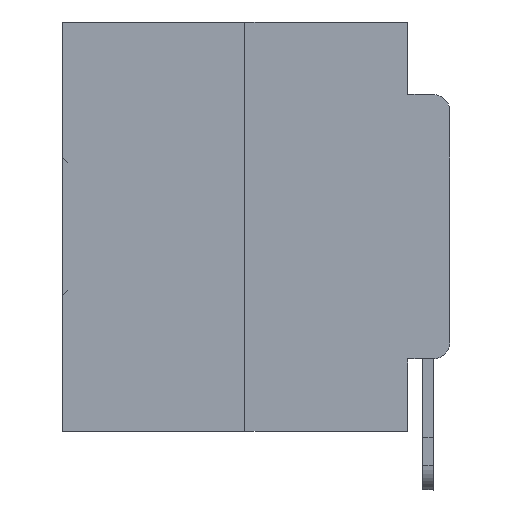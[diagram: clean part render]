
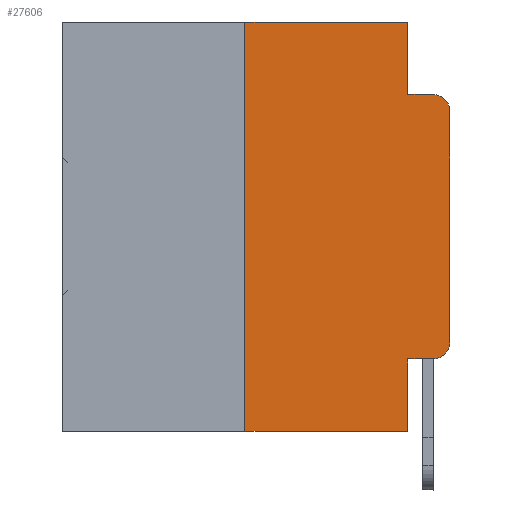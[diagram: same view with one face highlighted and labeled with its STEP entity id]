
A CAD part, left-side view. The second image highlights one B-rep face of the part: STEP entity #27606.
In plain terms, the highlighted planar face has unit normal (-1, 0, 0).
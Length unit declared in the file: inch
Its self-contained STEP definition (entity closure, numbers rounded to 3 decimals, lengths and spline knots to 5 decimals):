
#141 = VECTOR ( 'NONE', #23862, 39.37008 ) ;
#865 = DIRECTION ( 'NONE',  ( 0., 0., -1. ) ) ;
#1209 = DIRECTION ( 'NONE',  ( -1., 0., 0. ) ) ;
#1363 = CIRCLE ( 'NONE', #23575, 0.02 ) ;
#1619 = CARTESIAN_POINT ( 'NONE',  ( 0., 0.051, -0.0885 ) ) ;
#1834 = CIRCLE ( 'NONE', #33143, 0.02 ) ;
#2129 = CARTESIAN_POINT ( 'NONE',  ( 0., 0., 0. ) ) ;
#2879 = CARTESIAN_POINT ( 'NONE',  ( 0., 0.051, -0.4115 ) ) ;
#3120 = DIRECTION ( 'NONE',  ( 0., 0., -1. ) ) ;
#3246 = CARTESIAN_POINT ( 'NONE',  ( 0., 0.051, -0.0885 ) ) ;
#3296 = CARTESIAN_POINT ( 'NONE',  ( 0., 0.051, 0. ) ) ;
#3659 = ORIENTED_EDGE ( 'NONE', *, *, #18028, .T. ) ;
#4959 = CARTESIAN_POINT ( 'NONE',  ( 0., 0.473, 0. ) ) ;
#5288 = VERTEX_POINT ( 'NONE', #21463 ) ;
#6459 = DIRECTION ( 'NONE',  ( 0., 0., -1. ) ) ;
#7789 = CARTESIAN_POINT ( 'NONE',  ( 0., 0., -0.3915 ) ) ;
#7811 = DIRECTION ( 'NONE',  ( 0., -1., 0. ) ) ;
#8463 = CARTESIAN_POINT ( 'NONE',  ( 0., 0.02, -0.1085 ) ) ;
#8657 = CARTESIAN_POINT ( 'NONE',  ( 0., 0.051, 0. ) ) ;
#9633 = EDGE_CURVE ( 'NONE', #25301, #13045, #17312, .T. ) ;
#9908 = VERTEX_POINT ( 'NONE', #2879 ) ;
#10142 = LINE ( 'NONE', #4959, #20189 ) ;
#10471 = ORIENTED_EDGE ( 'NONE', *, *, #30483, .T. ) ;
#10658 = DIRECTION ( 'NONE',  ( 0., 0., -1. ) ) ;
#10670 = VERTEX_POINT ( 'NONE', #12458 ) ;
#10881 = CARTESIAN_POINT ( 'NONE',  ( 0., 0.02, -0.4115 ) ) ;
#12458 = CARTESIAN_POINT ( 'NONE',  ( 0., 0.051, -0.5 ) ) ;
#12841 = CARTESIAN_POINT ( 'NONE',  ( 0., 0.473, -0.5 ) ) ;
#13045 = VERTEX_POINT ( 'NONE', #3246 ) ;
#13111 = VECTOR ( 'NONE', #34380, 39.37008 ) ;
#13799 = VERTEX_POINT ( 'NONE', #24389 ) ;
#14133 = VECTOR ( 'NONE', #6459, 39.37008 ) ;
#14372 = LINE ( 'NONE', #17373, #21502 ) ;
#15102 = PLANE ( 'NONE',  #28408 ) ;
#15560 = EDGE_CURVE ( 'NONE', #17099, #33719, #1363, .T. ) ;
#15629 = DIRECTION ( 'NONE',  ( 1., 0., 0. ) ) ;
#15761 = CARTESIAN_POINT ( 'NONE',  ( 0., 0., -0.1085 ) ) ;
#15958 = ORIENTED_EDGE ( 'NONE', *, *, #29624, .F. ) ;
#17099 = VERTEX_POINT ( 'NONE', #15761 ) ;
#17312 = LINE ( 'NONE', #25520, #14133 ) ;
#17341 = EDGE_LOOP ( 'NONE', ( #35216, #27452, #32377, #30621, #17968, #20952, #10471, #15958, #3659, #30304 ) ) ;
#17373 = CARTESIAN_POINT ( 'NONE',  ( 0., 0.051, -0.4115 ) ) ;
#17394 = EDGE_CURVE ( 'NONE', #5288, #13799, #29043, .T. ) ;
#17822 = DIRECTION ( 'NONE',  ( 0., 0., 1. ) ) ;
#17968 = ORIENTED_EDGE ( 'NONE', *, *, #34623, .F. ) ;
#18028 = EDGE_CURVE ( 'NONE', #9908, #21316, #14372, .T. ) ;
#18310 = CARTESIAN_POINT ( 'NONE',  ( 0., 0.473, 0. ) ) ;
#19502 = LINE ( 'NONE', #3296, #29674 ) ;
#19892 = EDGE_CURVE ( 'NONE', #27723, #17099, #23333, .T. ) ;
#19914 = CARTESIAN_POINT ( 'NONE',  ( 0., 0.02, -0.3915 ) ) ;
#20189 = VECTOR ( 'NONE', #7811, 39.37008 ) ;
#20838 = CARTESIAN_POINT ( 'NONE',  ( 0., 0.25, 0. ) ) ;
#20952 = ORIENTED_EDGE ( 'NONE', *, *, #17394, .F. ) ;
#21316 = VERTEX_POINT ( 'NONE', #10881 ) ;
#21463 = CARTESIAN_POINT ( 'NONE',  ( 0., 0.25, -0.5 ) ) ;
#21502 = VECTOR ( 'NONE', #33086, 39.37008 ) ;
#22101 = VECTOR ( 'NONE', #17822, 39.37008 ) ;
#22741 = EDGE_CURVE ( 'NONE', #21316, #27723, #1834, .T. ) ;
#22992 = VECTOR ( 'NONE', #23175, 39.37008 ) ;
#23175 = DIRECTION ( 'NONE',  ( 0., -1., 0. ) ) ;
#23333 = LINE ( 'NONE', #2129, #13111 ) ;
#23575 = AXIS2_PLACEMENT_3D ( 'NONE', #8463, #30193, #27524 ) ;
#23685 = LINE ( 'NONE', #12841, #141 ) ;
#23862 = DIRECTION ( 'NONE',  ( 0., -1., 0. ) ) ;
#24389 = CARTESIAN_POINT ( 'NONE',  ( 0., 0.25, 0. ) ) ;
#25301 = VERTEX_POINT ( 'NONE', #8657 ) ;
#25520 = CARTESIAN_POINT ( 'NONE',  ( 0., 0.051, 0. ) ) ;
#27452 = ORIENTED_EDGE ( 'NONE', *, *, #15560, .T. ) ;
#27524 = DIRECTION ( 'NONE',  ( 0., 0., -1. ) ) ;
#27606 = ADVANCED_FACE ( 'NONE', ( #31861 ), #15102, .F. ) ;
#27723 = VERTEX_POINT ( 'NONE', #7789 ) ;
#28408 = AXIS2_PLACEMENT_3D ( 'NONE', #18310, #15629, #10658 ) ;
#29043 = LINE ( 'NONE', #20838, #22101 ) ;
#29624 = EDGE_CURVE ( 'NONE', #9908, #10670, #19502, .T. ) ;
#29674 = VECTOR ( 'NONE', #3120, 39.37008 ) ;
#30193 = DIRECTION ( 'NONE',  ( -1., 0., 0. ) ) ;
#30304 = ORIENTED_EDGE ( 'NONE', *, *, #22741, .T. ) ;
#30483 = EDGE_CURVE ( 'NONE', #5288, #10670, #23685, .T. ) ;
#30621 = ORIENTED_EDGE ( 'NONE', *, *, #9633, .F. ) ;
#31861 = FACE_OUTER_BOUND ( 'NONE', #17341, .T. ) ;
#32377 = ORIENTED_EDGE ( 'NONE', *, *, #34062, .F. ) ;
#33086 = DIRECTION ( 'NONE',  ( 0., -1., 0. ) ) ;
#33143 = AXIS2_PLACEMENT_3D ( 'NONE', #19914, #1209, #865 ) ;
#33719 = VERTEX_POINT ( 'NONE', #34452 ) ;
#33860 = LINE ( 'NONE', #1619, #22992 ) ;
#34062 = EDGE_CURVE ( 'NONE', #13045, #33719, #33860, .T. ) ;
#34380 = DIRECTION ( 'NONE',  ( 0., 0., 1. ) ) ;
#34452 = CARTESIAN_POINT ( 'NONE',  ( 0., 0.02, -0.0885 ) ) ;
#34623 = EDGE_CURVE ( 'NONE', #13799, #25301, #10142, .T. ) ;
#35216 = ORIENTED_EDGE ( 'NONE', *, *, #19892, .T. ) ;
